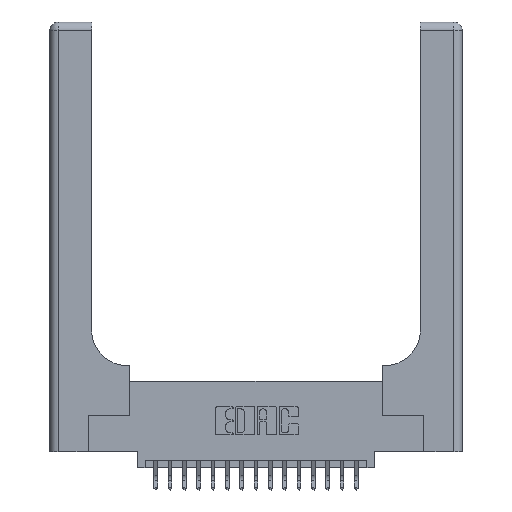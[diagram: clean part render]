
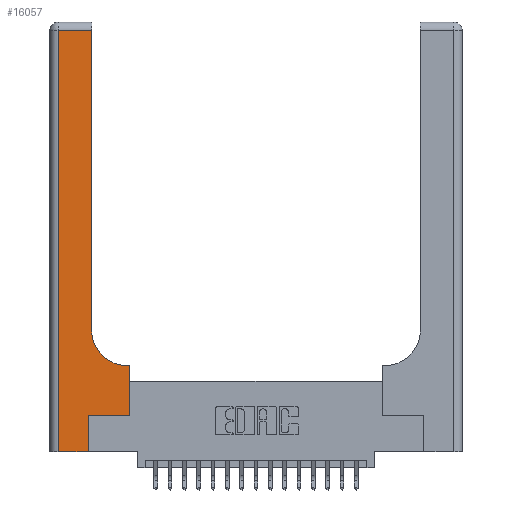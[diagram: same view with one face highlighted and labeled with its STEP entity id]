
A CAD part, top view. The second image highlights one B-rep face of the part: STEP entity #16057.
In plain terms, the highlighted planar face has unit normal (0, 0, 1).
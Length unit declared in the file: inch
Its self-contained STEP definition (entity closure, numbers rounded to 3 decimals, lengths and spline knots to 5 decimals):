
#101 = CARTESIAN_POINT ( 'NONE',  ( 0.2915, 0.85, 0.37 ) ) ;
#454 = CARTESIAN_POINT ( 'NONE',  ( 0.269, 0., 0.37 ) ) ;
#475 = PLANE ( 'NONE',  #15339 ) ;
#689 = EDGE_CURVE ( 'NONE', #19229, #13081, #13280, .T. ) ;
#928 = VECTOR ( 'NONE', #955, 39.37008 ) ;
#955 = DIRECTION ( 'NONE',  ( -1., 0., 0. ) ) ;
#1226 = EDGE_CURVE ( 'NONE', #6092, #19229, #16969, .T. ) ;
#1407 = DIRECTION ( 'NONE',  ( 0., -1., 0. ) ) ;
#1463 = CARTESIAN_POINT ( 'NONE',  ( 0.5585, 0.25, 0.37 ) ) ;
#1673 = EDGE_CURVE ( 'NONE', #20038, #10508, #13245, .T. ) ;
#1689 = ORIENTED_EDGE ( 'NONE', *, *, #1673, .T. ) ;
#1737 = DIRECTION ( 'NONE',  ( 0., 1., 0. ) ) ;
#1801 = CARTESIAN_POINT ( 'NONE',  ( 0.269, 0., 0.37 ) ) ;
#2401 = ORIENTED_EDGE ( 'NONE', *, *, #689, .T. ) ;
#2657 = VECTOR ( 'NONE', #1407, 39.37008 ) ;
#3142 = VERTEX_POINT ( 'NONE', #9280 ) ;
#3187 = VECTOR ( 'NONE', #10819, 39.37008 ) ;
#3215 = VECTOR ( 'NONE', #6651, 39.37008 ) ;
#3868 = DIRECTION ( 'NONE',  ( -1., 0., 0. ) ) ;
#4515 = CARTESIAN_POINT ( 'NONE',  ( 0.269, 0.25, 0.37 ) ) ;
#4594 = ORIENTED_EDGE ( 'NONE', *, *, #18801, .T. ) ;
#4631 = CARTESIAN_POINT ( 'NONE',  ( 0.06, 2.94, 0.37 ) ) ;
#4692 = CARTESIAN_POINT ( 'NONE',  ( 0.5585, 0.6, 0.37 ) ) ;
#5668 = VERTEX_POINT ( 'NONE', #101 ) ;
#5918 = CARTESIAN_POINT ( 'NONE',  ( 0.2915, 3., 0.37 ) ) ;
#6092 = VERTEX_POINT ( 'NONE', #11241 ) ;
#6443 = CARTESIAN_POINT ( 'NONE',  ( 0.06, 3., 0.37 ) ) ;
#6651 = DIRECTION ( 'NONE',  ( 1., 0., 0. ) ) ;
#6688 = LINE ( 'NONE', #15048, #14692 ) ;
#7596 = DIRECTION ( 'NONE',  ( 0., 1., 0. ) ) ;
#7643 = CARTESIAN_POINT ( 'NONE',  ( 0.5415, 0.6, 0.37 ) ) ;
#7669 = LINE ( 'NONE', #9800, #3215 ) ;
#7724 = ORIENTED_EDGE ( 'NONE', *, *, #13865, .T. ) ;
#7970 = CARTESIAN_POINT ( 'NONE',  ( 0.5585, 0.25, 0.37 ) ) ;
#8133 = ORIENTED_EDGE ( 'NONE', *, *, #1226, .T. ) ;
#8634 = LINE ( 'NONE', #5918, #3187 ) ;
#8686 = DIRECTION ( 'NONE',  ( -1., 0., 0. ) ) ;
#8786 = CARTESIAN_POINT ( 'NONE',  ( 0., 3., 0.37 ) ) ;
#8981 = VECTOR ( 'NONE', #7596, 39.37008 ) ;
#9013 = VECTOR ( 'NONE', #1737, 39.37008 ) ;
#9280 = CARTESIAN_POINT ( 'NONE',  ( 0.2915, 2.94, 0.37 ) ) ;
#9505 = CARTESIAN_POINT ( 'NONE',  ( 0.5415, 0.85, 0.37 ) ) ;
#9794 = VERTEX_POINT ( 'NONE', #7643 ) ;
#9800 = CARTESIAN_POINT ( 'NONE',  ( 0.269, 0.25, 0.37 ) ) ;
#9812 = CIRCLE ( 'NONE', #12166, 0.25 ) ;
#10508 = VERTEX_POINT ( 'NONE', #4692 ) ;
#10819 = DIRECTION ( 'NONE',  ( 0., 1., 0. ) ) ;
#11132 = DIRECTION ( 'NONE',  ( 1., 0., 0. ) ) ;
#11241 = CARTESIAN_POINT ( 'NONE',  ( 0.06, 0., 0.37 ) ) ;
#12166 = AXIS2_PLACEMENT_3D ( 'NONE', #9505, #20559, #11132 ) ;
#12757 = VECTOR ( 'NONE', #14759, 39.37008 ) ;
#12896 = EDGE_LOOP ( 'NONE', ( #14493, #20969, #15113, #8133, #2401, #7724, #1689, #15589, #4594 ) ) ;
#13081 = VERTEX_POINT ( 'NONE', #4515 ) ;
#13245 = LINE ( 'NONE', #7970, #8981 ) ;
#13280 = LINE ( 'NONE', #1801, #9013 ) ;
#13459 = EDGE_CURVE ( 'NONE', #3142, #13807, #6688, .T. ) ;
#13616 = DIRECTION ( 'NONE',  ( 0., 0., -1. ) ) ;
#13807 = VERTEX_POINT ( 'NONE', #4631 ) ;
#13865 = EDGE_CURVE ( 'NONE', #13081, #20038, #7669, .T. ) ;
#13995 = LINE ( 'NONE', #20316, #928 ) ;
#14493 = ORIENTED_EDGE ( 'NONE', *, *, #16761, .T. ) ;
#14692 = VECTOR ( 'NONE', #8686, 39.37008 ) ;
#14759 = DIRECTION ( 'NONE',  ( 1., 0., 0. ) ) ;
#14802 = CARTESIAN_POINT ( 'NONE',  ( 0., 0., 0.37 ) ) ;
#15048 = CARTESIAN_POINT ( 'NONE',  ( 0., 2.94, 0.37 ) ) ;
#15081 = EDGE_CURVE ( 'NONE', #13807, #6092, #19562, .T. ) ;
#15113 = ORIENTED_EDGE ( 'NONE', *, *, #15081, .T. ) ;
#15339 = AXIS2_PLACEMENT_3D ( 'NONE', #8786, #13616, #3868 ) ;
#15589 = ORIENTED_EDGE ( 'NONE', *, *, #20849, .T. ) ;
#16057 = ADVANCED_FACE ( 'NONE', ( #16888 ), #475, .F. ) ;
#16761 = EDGE_CURVE ( 'NONE', #5668, #3142, #8634, .T. ) ;
#16888 = FACE_OUTER_BOUND ( 'NONE', #12896, .T. ) ;
#16969 = LINE ( 'NONE', #14802, #12757 ) ;
#18801 = EDGE_CURVE ( 'NONE', #9794, #5668, #9812, .T. ) ;
#19229 = VERTEX_POINT ( 'NONE', #454 ) ;
#19562 = LINE ( 'NONE', #6443, #2657 ) ;
#20038 = VERTEX_POINT ( 'NONE', #1463 ) ;
#20316 = CARTESIAN_POINT ( 'NONE',  ( 0.2915, 0.6, 0.37 ) ) ;
#20559 = DIRECTION ( 'NONE',  ( 0., 0., -1. ) ) ;
#20849 = EDGE_CURVE ( 'NONE', #10508, #9794, #13995, .T. ) ;
#20969 = ORIENTED_EDGE ( 'NONE', *, *, #13459, .T. ) ;
